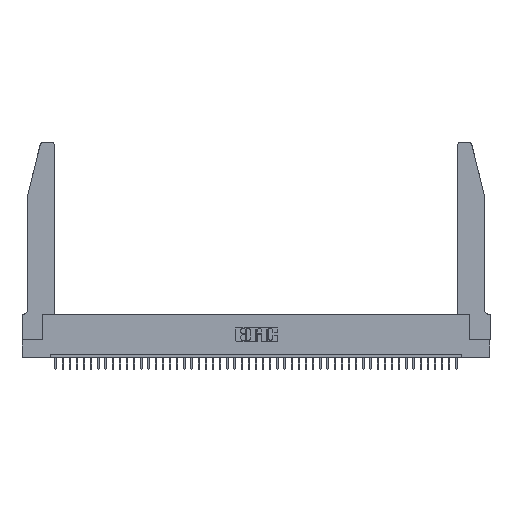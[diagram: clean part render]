
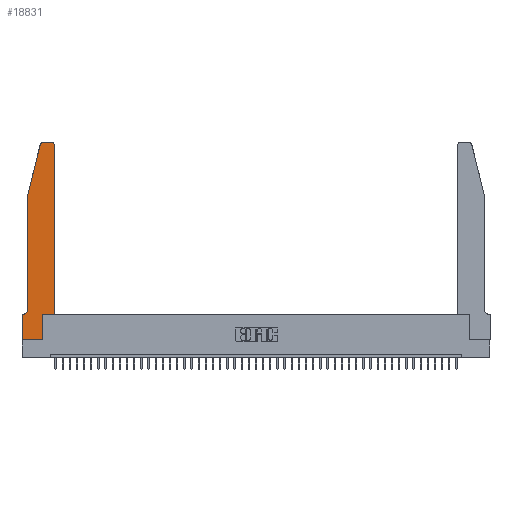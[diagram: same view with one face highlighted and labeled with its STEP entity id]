
A CAD part, top view. The second image highlights one B-rep face of the part: STEP entity #18831.
In plain terms, the highlighted planar face has unit normal (0, 0, 1).
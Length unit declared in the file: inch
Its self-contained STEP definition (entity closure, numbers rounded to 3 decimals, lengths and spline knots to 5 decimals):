
#192 = LINE ( 'NONE', #16671, #39367 ) ;
#1361 = DIRECTION ( 'NONE',  ( 1., 0., 0. ) ) ;
#1415 = DIRECTION ( 'NONE',  ( 0., 0., 1. ) ) ;
#2623 = CARTESIAN_POINT ( 'NONE',  ( 0.0055, 0.42, 0.37 ) ) ;
#2676 = LINE ( 'NONE', #38642, #29763 ) ;
#2822 = VERTEX_POINT ( 'NONE', #24191 ) ;
#4129 = LINE ( 'NONE', #23115, #14098 ) ;
#4519 = EDGE_CURVE ( 'NONE', #37936, #2822, #27118, .T. ) ;
#5348 = LINE ( 'NONE', #22507, #36244 ) ;
#5470 = AXIS2_PLACEMENT_3D ( 'NONE', #43157, #6931, #8128 ) ;
#5560 = DIRECTION ( 'NONE',  ( 0., 0., -1. ) ) ;
#5599 = CARTESIAN_POINT ( 'NONE',  ( 0.0055, 0.35, 0.37 ) ) ;
#5645 = CARTESIAN_POINT ( 'NONE',  ( 0.2865, 0., 0.37 ) ) ;
#5868 = DIRECTION ( 'NONE',  ( 1., 0., 0. ) ) ;
#6593 = VERTEX_POINT ( 'NONE', #11448 ) ;
#6931 = DIRECTION ( 'NONE',  ( 0., 0., 1. ) ) ;
#7663 = LINE ( 'NONE', #32635, #14335 ) ;
#8128 = DIRECTION ( 'NONE',  ( 1., 0., 0. ) ) ;
#8849 = VERTEX_POINT ( 'NONE', #26831 ) ;
#9258 = EDGE_CURVE ( 'NONE', #41452, #6593, #2676, .T. ) ;
#10008 = PLANE ( 'NONE',  #31984 ) ;
#10337 = EDGE_CURVE ( 'NONE', #28656, #30383, #21317, .T. ) ;
#10537 = ORIENTED_EDGE ( 'NONE', *, *, #10337, .T. ) ;
#11012 = EDGE_CURVE ( 'NONE', #2822, #44614, #25591, .T. ) ;
#11448 = CARTESIAN_POINT ( 'NONE',  ( 0.4505, 2.72, 0.37 ) ) ;
#12601 = EDGE_CURVE ( 'NONE', #6593, #44876, #38641, .T. ) ;
#13790 = EDGE_CURVE ( 'NONE', #30383, #41452, #5348, .T. ) ;
#14098 = VECTOR ( 'NONE', #5868, 39.37008 ) ;
#14335 = VECTOR ( 'NONE', #39676, 39.37008 ) ;
#14689 = ORIENTED_EDGE ( 'NONE', *, *, #9258, .T. ) ;
#15059 = EDGE_CURVE ( 'NONE', #23440, #27759, #41749, .T. ) ;
#15579 = CARTESIAN_POINT ( 'NONE',  ( 0.284, 2.75, 0.37 ) ) ;
#16182 = DIRECTION ( 'NONE',  ( -1., 0., 0. ) ) ;
#16671 = CARTESIAN_POINT ( 'NONE',  ( 0., 0., 0.37 ) ) ;
#17073 = CARTESIAN_POINT ( 'NONE',  ( 0., 0.35, 0.37 ) ) ;
#17537 = DIRECTION ( 'NONE',  ( 0., 0., 1. ) ) ;
#18006 = VECTOR ( 'NONE', #29840, 39.37008 ) ;
#18386 = CARTESIAN_POINT ( 'NONE',  ( 0., 0.35, 0.37 ) ) ;
#18831 = ADVANCED_FACE ( 'NONE', ( #29615 ), #10008, .T. ) ;
#19169 = EDGE_CURVE ( 'NONE', #8849, #28656, #4129, .T. ) ;
#20930 = ORIENTED_EDGE ( 'NONE', *, *, #4519, .T. ) ;
#21317 = LINE ( 'NONE', #37844, #26827 ) ;
#21569 = DIRECTION ( 'NONE',  ( -0.239, -0.971, 0. ) ) ;
#21926 = AXIS2_PLACEMENT_3D ( 'NONE', #2623, #5560, #16182 ) ;
#22092 = VECTOR ( 'NONE', #45628, 39.37008 ) ;
#22449 = ORIENTED_EDGE ( 'NONE', *, *, #13790, .T. ) ;
#22507 = CARTESIAN_POINT ( 'NONE',  ( 0.4505, 0.35, 0.37 ) ) ;
#22775 = CARTESIAN_POINT ( 'NONE',  ( 0.2865, 0.35, 0.37 ) ) ;
#23115 = CARTESIAN_POINT ( 'NONE',  ( 0., 0., 0.37 ) ) ;
#23440 = VERTEX_POINT ( 'NONE', #15579 ) ;
#23517 = EDGE_CURVE ( 'NONE', #27759, #37936, #38580, .T. ) ;
#23916 = ORIENTED_EDGE ( 'NONE', *, *, #23517, .T. ) ;
#24191 = CARTESIAN_POINT ( 'NONE',  ( 0.0755, 0.42, 0.37 ) ) ;
#25268 = CARTESIAN_POINT ( 'NONE',  ( 0.4205, 2.75, 0.37 ) ) ;
#25591 = CIRCLE ( 'NONE', #21926, 0.07 ) ;
#26161 = ORIENTED_EDGE ( 'NONE', *, *, #12601, .T. ) ;
#26827 = VECTOR ( 'NONE', #41392, 39.37008 ) ;
#26831 = CARTESIAN_POINT ( 'NONE',  ( 0., 0., 0.37 ) ) ;
#27118 = LINE ( 'NONE', #35304, #22092 ) ;
#27759 = VERTEX_POINT ( 'NONE', #36592 ) ;
#27822 = DIRECTION ( 'NONE',  ( 0., -1., 0. ) ) ;
#28076 = DIRECTION ( 'NONE',  ( 1., 0., 0. ) ) ;
#28425 = CARTESIAN_POINT ( 'NONE',  ( 0.0755, 2., 0.37 ) ) ;
#28656 = VERTEX_POINT ( 'NONE', #5645 ) ;
#29615 = FACE_OUTER_BOUND ( 'NONE', #35580, .T. ) ;
#29710 = CARTESIAN_POINT ( 'NONE',  ( 0.0755, 2., 0.37 ) ) ;
#29763 = VECTOR ( 'NONE', #38175, 39.37008 ) ;
#29840 = DIRECTION ( 'NONE',  ( -1., 0., 0. ) ) ;
#30383 = VERTEX_POINT ( 'NONE', #22775 ) ;
#31316 = ORIENTED_EDGE ( 'NONE', *, *, #31531, .T. ) ;
#31322 = ORIENTED_EDGE ( 'NONE', *, *, #35632, .T. ) ;
#31531 = EDGE_CURVE ( 'NONE', #44614, #37864, #7663, .T. ) ;
#31546 = DIRECTION ( 'NONE',  ( 1., 0., 0. ) ) ;
#31984 = AXIS2_PLACEMENT_3D ( 'NONE', #17073, #17537, #28076 ) ;
#32635 = CARTESIAN_POINT ( 'NONE',  ( 0.0755, 0.35, 0.37 ) ) ;
#33368 = EDGE_CURVE ( 'NONE', #44876, #23440, #39022, .T. ) ;
#33802 = ORIENTED_EDGE ( 'NONE', *, *, #33368, .T. ) ;
#35304 = CARTESIAN_POINT ( 'NONE',  ( 0.0755, 2., 0.37 ) ) ;
#35580 = EDGE_LOOP ( 'NONE', ( #33802, #40322, #23916, #20930, #42572, #31316, #31322, #45354, #10537, #22449, #14689, #26161 ) ) ;
#35632 = EDGE_CURVE ( 'NONE', #37864, #8849, #192, .T. ) ;
#36244 = VECTOR ( 'NONE', #1361, 39.37008 ) ;
#36592 = CARTESIAN_POINT ( 'NONE',  ( 0.25487, 2.72718, 0.37 ) ) ;
#37453 = VECTOR ( 'NONE', #21569, 39.37008 ) ;
#37844 = CARTESIAN_POINT ( 'NONE',  ( 0.2865, 0.35, 0.37 ) ) ;
#37864 = VERTEX_POINT ( 'NONE', #18386 ) ;
#37901 = CARTESIAN_POINT ( 'NONE',  ( 0.2605, 2.75, 0.37 ) ) ;
#37936 = VERTEX_POINT ( 'NONE', #29710 ) ;
#38175 = DIRECTION ( 'NONE',  ( 0., 1., 0. ) ) ;
#38580 = LINE ( 'NONE', #28425, #37453 ) ;
#38641 = CIRCLE ( 'NONE', #44772, 0.03 ) ;
#38642 = CARTESIAN_POINT ( 'NONE',  ( 0.4505, 0.35, 0.37 ) ) ;
#38948 = CARTESIAN_POINT ( 'NONE',  ( 0.4505, 0.35, 0.37 ) ) ;
#39022 = LINE ( 'NONE', #37901, #18006 ) ;
#39367 = VECTOR ( 'NONE', #27822, 39.37008 ) ;
#39676 = DIRECTION ( 'NONE',  ( -1., 0., 0. ) ) ;
#40022 = CARTESIAN_POINT ( 'NONE',  ( 0.4205, 2.72, 0.37 ) ) ;
#40322 = ORIENTED_EDGE ( 'NONE', *, *, #15059, .T. ) ;
#41392 = DIRECTION ( 'NONE',  ( 0., 1., 0. ) ) ;
#41452 = VERTEX_POINT ( 'NONE', #38948 ) ;
#41749 = CIRCLE ( 'NONE', #5470, 0.03 ) ;
#42572 = ORIENTED_EDGE ( 'NONE', *, *, #11012, .T. ) ;
#43157 = CARTESIAN_POINT ( 'NONE',  ( 0.284, 2.72, 0.37 ) ) ;
#44614 = VERTEX_POINT ( 'NONE', #5599 ) ;
#44772 = AXIS2_PLACEMENT_3D ( 'NONE', #40022, #1415, #31546 ) ;
#44876 = VERTEX_POINT ( 'NONE', #25268 ) ;
#45354 = ORIENTED_EDGE ( 'NONE', *, *, #19169, .T. ) ;
#45628 = DIRECTION ( 'NONE',  ( 0., -1., 0. ) ) ;
